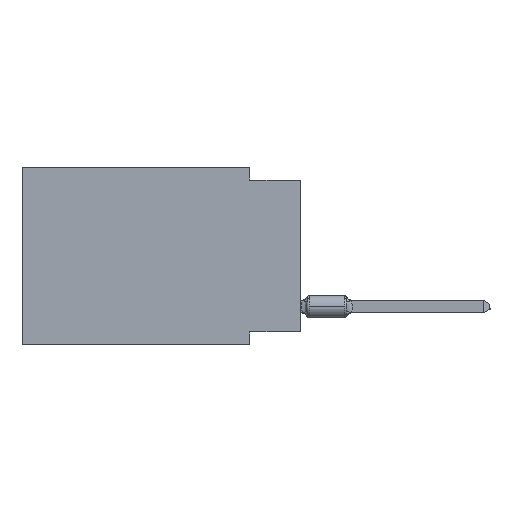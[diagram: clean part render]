
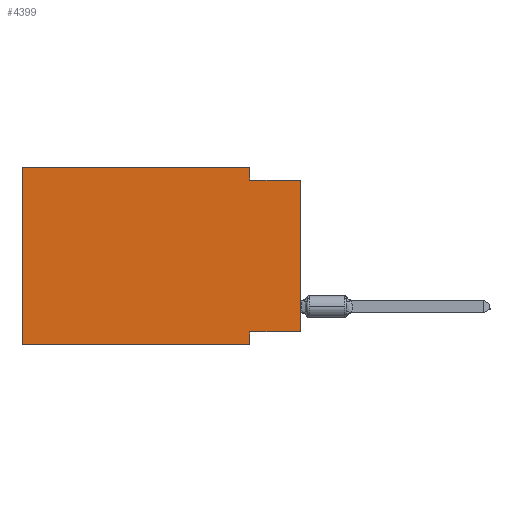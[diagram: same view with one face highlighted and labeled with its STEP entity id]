
A CAD part, left-side view. The second image highlights one B-rep face of the part: STEP entity #4399.
In plain terms, the highlighted planar face has unit normal (-1, 0, 0).
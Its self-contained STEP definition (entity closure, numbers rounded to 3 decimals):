
#310 = DIRECTION ( 'NONE',  ( 0., 1., 0. ) ) ;
#446 = ORIENTED_EDGE ( 'NONE', *, *, #40216, .T. ) ;
#1670 = CARTESIAN_POINT ( 'NONE',  ( 0., 0., -0.635 ) ) ;
#1693 = LINE ( 'NONE', #30264, #23278 ) ;
#1701 = CARTESIAN_POINT ( 'NONE',  ( 0., 2.54, -0.635 ) ) ;
#2320 = LINE ( 'NONE', #44808, #10154 ) ;
#2828 = VERTEX_POINT ( 'NONE', #1701 ) ;
#3223 = VECTOR ( 'NONE', #28037, 1000. ) ;
#4399 = ADVANCED_FACE ( 'NONE', ( #45674 ), #20397, .F. ) ;
#4524 = VECTOR ( 'NONE', #10883, 1000. ) ;
#4902 = ORIENTED_EDGE ( 'NONE', *, *, #34172, .F. ) ;
#5378 = CARTESIAN_POINT ( 'NONE',  ( 0., 2.54, 0. ) ) ;
#6434 = VECTOR ( 'NONE', #26773, 1000. ) ;
#6445 = CARTESIAN_POINT ( 'NONE',  ( 0., 13.97, 0. ) ) ;
#6616 = CARTESIAN_POINT ( 'NONE',  ( 0., 13.97, 0. ) ) ;
#7150 = CARTESIAN_POINT ( 'NONE',  ( 0., 2.54, -8.89 ) ) ;
#9065 = LINE ( 'NONE', #33676, #41330 ) ;
#9909 = VERTEX_POINT ( 'NONE', #10959 ) ;
#10037 = VECTOR ( 'NONE', #17081, 1000. ) ;
#10154 = VECTOR ( 'NONE', #310, 1000. ) ;
#10388 = LINE ( 'NONE', #27569, #3223 ) ;
#10883 = DIRECTION ( 'NONE',  ( 0., 0., -1. ) ) ;
#10959 = CARTESIAN_POINT ( 'NONE',  ( 0., 2.54, -8.89 ) ) ;
#13741 = VERTEX_POINT ( 'NONE', #1670 ) ;
#14986 = VERTEX_POINT ( 'NONE', #5378 ) ;
#16133 = ORIENTED_EDGE ( 'NONE', *, *, #41770, .F. ) ;
#16333 = ORIENTED_EDGE ( 'NONE', *, *, #18906, .F. ) ;
#17081 = DIRECTION ( 'NONE',  ( 0., -1., 0. ) ) ;
#17445 = ORIENTED_EDGE ( 'NONE', *, *, #29314, .F. ) ;
#18068 = LINE ( 'NONE', #7150, #4524 ) ;
#18725 = CARTESIAN_POINT ( 'NONE',  ( 0., 13.97, -8.89 ) ) ;
#18906 = EDGE_CURVE ( 'NONE', #22468, #32131, #2320, .T. ) ;
#20092 = LINE ( 'NONE', #6616, #10037 ) ;
#20397 = PLANE ( 'NONE',  #29659 ) ;
#20962 = EDGE_CURVE ( 'NONE', #32131, #9909, #18068, .T. ) ;
#21289 = CARTESIAN_POINT ( 'NONE',  ( 0., 2.54, -8.255 ) ) ;
#21541 = LINE ( 'NONE', #18725, #39241 ) ;
#22468 = VERTEX_POINT ( 'NONE', #44044 ) ;
#22982 = VERTEX_POINT ( 'NONE', #38036 ) ;
#23240 = DIRECTION ( 'NONE',  ( 0., 0., 1. ) ) ;
#23278 = VECTOR ( 'NONE', #23304, 1000. ) ;
#23304 = DIRECTION ( 'NONE',  ( 0., 0., -1. ) ) ;
#25663 = EDGE_CURVE ( 'NONE', #22468, #13741, #10388, .T. ) ;
#26773 = DIRECTION ( 'NONE',  ( 0., -1., 0. ) ) ;
#27073 = EDGE_CURVE ( 'NONE', #30818, #14986, #20092, .T. ) ;
#27079 = EDGE_LOOP ( 'NONE', ( #43565, #16133, #4902, #28817, #17445, #446, #27145, #16333 ) ) ;
#27145 = ORIENTED_EDGE ( 'NONE', *, *, #20962, .F. ) ;
#27569 = CARTESIAN_POINT ( 'NONE',  ( 0., 0., 0. ) ) ;
#28037 = DIRECTION ( 'NONE',  ( 0., 0., 1. ) ) ;
#28817 = ORIENTED_EDGE ( 'NONE', *, *, #27073, .F. ) ;
#29174 = CARTESIAN_POINT ( 'NONE',  ( 0., 0., -0.635 ) ) ;
#29314 = EDGE_CURVE ( 'NONE', #22982, #30818, #9065, .T. ) ;
#29659 = AXIS2_PLACEMENT_3D ( 'NONE', #6445, #41731, #34777 ) ;
#30264 = CARTESIAN_POINT ( 'NONE',  ( 0., 2.54, 0. ) ) ;
#30818 = VERTEX_POINT ( 'NONE', #44259 ) ;
#32131 = VERTEX_POINT ( 'NONE', #21289 ) ;
#32660 = DIRECTION ( 'NONE',  ( 0., -1., 0. ) ) ;
#33676 = CARTESIAN_POINT ( 'NONE',  ( 0., 13.97, 0. ) ) ;
#34172 = EDGE_CURVE ( 'NONE', #14986, #2828, #1693, .T. ) ;
#34777 = DIRECTION ( 'NONE',  ( 0., 0., -1. ) ) ;
#38036 = CARTESIAN_POINT ( 'NONE',  ( 0., 13.97, -8.89 ) ) ;
#39241 = VECTOR ( 'NONE', #32660, 1000. ) ;
#40216 = EDGE_CURVE ( 'NONE', #22982, #9909, #21541, .T. ) ;
#41150 = LINE ( 'NONE', #29174, #6434 ) ;
#41330 = VECTOR ( 'NONE', #23240, 1000. ) ;
#41731 = DIRECTION ( 'NONE',  ( 1., 0., 0. ) ) ;
#41770 = EDGE_CURVE ( 'NONE', #2828, #13741, #41150, .T. ) ;
#43565 = ORIENTED_EDGE ( 'NONE', *, *, #25663, .T. ) ;
#44044 = CARTESIAN_POINT ( 'NONE',  ( 0., 0., -8.255 ) ) ;
#44259 = CARTESIAN_POINT ( 'NONE',  ( 0., 13.97, 0. ) ) ;
#44808 = CARTESIAN_POINT ( 'NONE',  ( 0., 0., -8.255 ) ) ;
#45674 = FACE_OUTER_BOUND ( 'NONE', #27079, .T. ) ;
